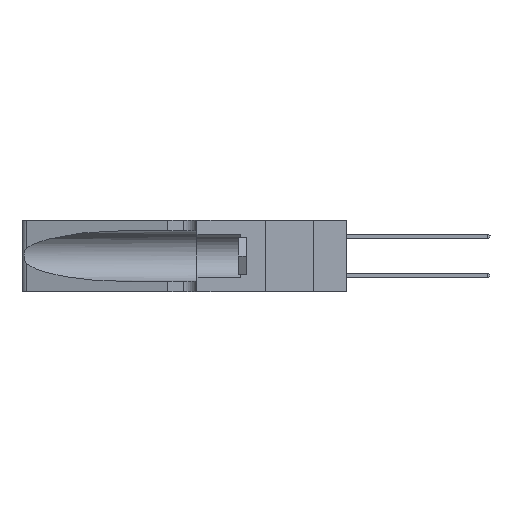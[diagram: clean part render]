
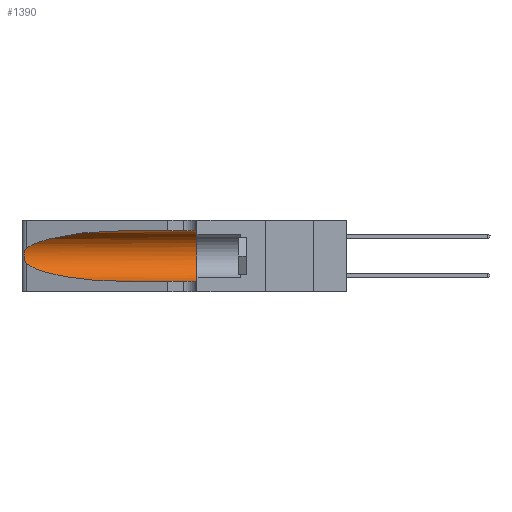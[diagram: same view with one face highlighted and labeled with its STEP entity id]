
A CAD part, left-side view. The second image highlights one B-rep face of the part: STEP entity #1390.
In plain terms, the highlighted cylindrical face has radius 3.308 mm (diameter 6.617 mm), a partial arc.
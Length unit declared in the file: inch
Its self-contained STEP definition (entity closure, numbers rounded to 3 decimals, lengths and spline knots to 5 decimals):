
#110 = CARTESIAN_POINT ( 'NONE',  ( 0.26075, 1.23896, 0.178 ) ) ;
#476 = CARTESIAN_POINT ( 'NONE',  ( 0.2373, 1.15595, 0.28018 ) ) ;
#1249 = LINE ( 'NONE', #17443, #2117 ) ;
#1390 = ADVANCED_FACE ( 'NONE', ( #17853 ), #30696, .F. ) ;
#1551 = DIRECTION ( 'NONE',  ( 0., -1., 0. ) ) ;
#2117 = VECTOR ( 'NONE', #9579, 39.37008 ) ;
#2698 = VECTOR ( 'NONE', #1551, 39.37008 ) ;
#2896 = CARTESIAN_POINT ( 'NONE',  ( 0.25856, 1.23593, 0.16098 ) ) ;
#3001 = CARTESIAN_POINT ( 'NONE',  ( 0.25487, 1.22718, 0.22369 ) ) ;
#3516 = VERTEX_POINT ( 'NONE', #25583 ) ;
#5539 = CARTESIAN_POINT ( 'NONE',  ( 0.25555, 1.22994, 0.2215 ) ) ;
#5658 = CARTESIAN_POINT ( 'NONE',  ( 0.25639, 1.23186, 0.15144 ) ) ;
#7256 = CARTESIAN_POINT ( 'NONE',  ( 0.1305, 0.72297, 0.05475 ) ) ;
#7417 = ORIENTED_EDGE ( 'NONE', *, *, #27692, .T. ) ;
#8304 = CARTESIAN_POINT ( 'NONE',  ( 0.25487, 1.22718, 0.14631 ) ) ;
#8323 = VERTEX_POINT ( 'NONE', #11542 ) ;
#8373 = CARTESIAN_POINT ( 'NONE',  ( 0.25487, 1.22718, 0.14631 ) ) ;
#8533 = B_SPLINE_CURVE_WITH_KNOTS ( 'NONE', 3,
 ( #23815, #5539, #10922, #28944, #13513, #31569, #16165, #110, #18783, #2896, #21352, #5658, #23934, #8373 ),
 .UNSPECIFIED., .F., .F.,
 ( 4, 2, 2, 2, 2, 2, 4 ),
 ( 0., 0.00027, 0.00053, 0.00107, 0.0016, 0.00187, 0.00214 ),
 .UNSPECIFIED. ) ;
#9547 = CIRCLE ( 'NONE', #22199, 0.13025 ) ;
#9579 = DIRECTION ( 'NONE',  ( 0., -1., 0. ) ) ;
#10688 = CARTESIAN_POINT ( 'NONE',  ( 0.1305, 0.35, 0.185 ) ) ;
#10922 = CARTESIAN_POINT ( 'NONE',  ( 0.25639, 1.23184, 0.21858 ) ) ;
#10957 = CARTESIAN_POINT ( 'NONE',  ( 0.18966, 0.96281, 0.05475 ) ) ;
#11426 = ORIENTED_EDGE ( 'NONE', *, *, #33828, .F. ) ;
#11542 = CARTESIAN_POINT ( 'NONE',  ( 0.1305, 0.35, 0.31525 ) ) ;
#11917 = VERTEX_POINT ( 'NONE', #7256 ) ;
#13269 = DIRECTION ( 'NONE',  ( 0., 0., 1. ) ) ;
#13513 = CARTESIAN_POINT ( 'NONE',  ( 0.25854, 1.2359, 0.20912 ) ) ;
#13858 = CARTESIAN_POINT ( 'NONE',  ( 0.1305, 0.72297, 0.31525 ) ) ;
#14127 = EDGE_CURVE ( 'NONE', #11917, #20566, #1249, .T. ) ;
#15168 = DIRECTION ( 'NONE',  ( 0., -1., 0. ) ) ;
#15667 = EDGE_LOOP ( 'NONE', ( #7417, #26430, #25985, #16263, #27397, #11426 ) ) ;
#16102 = CARTESIAN_POINT ( 'NONE',  ( 0.2373, 1.15595, 0.08982 ) ) ;
#16165 = CARTESIAN_POINT ( 'NONE',  ( 0.26075, 1.23896, 0.19203 ) ) ;
#16263 = ORIENTED_EDGE ( 'NONE', *, *, #14127, .T. ) ;
#16501 = CARTESIAN_POINT ( 'NONE',  ( 0.18966, 0.96281, 0.31525 ) ) ;
#17443 = CARTESIAN_POINT ( 'NONE',  ( 0.1305, 1.61858, 0.05475 ) ) ;
#17853 = FACE_OUTER_BOUND ( 'NONE', #15667, .T. ) ;
#18157 =( BOUNDED_CURVE ( )  B_SPLINE_CURVE ( 3, ( #13858, #16501, #476, #19125 ),
 .UNSPECIFIED., .F., .F. ) 
 B_SPLINE_CURVE_WITH_KNOTS ( ( 4, 4 ),
 ( 1.5708, 2.84003 ),
 .UNSPECIFIED. ) 
 CURVE ( )  GEOMETRIC_REPRESENTATION_ITEM ( )  RATIONAL_B_SPLINE_CURVE ( ( 1., 0.87, 0.87, 1. ) ) 
 REPRESENTATION_ITEM ( '' )  );
#18484 = LINE ( 'NONE', #30299, #2698 ) ;
#18783 = CARTESIAN_POINT ( 'NONE',  ( 0.26017, 1.23833, 0.17102 ) ) ;
#19125 = CARTESIAN_POINT ( 'NONE',  ( 0.25487, 1.22718, 0.22369 ) ) ;
#20566 = VERTEX_POINT ( 'NONE', #26972 ) ;
#20776 = AXIS2_PLACEMENT_3D ( 'NONE', #33074, #15168, #22849 ) ;
#21032 = EDGE_CURVE ( 'NONE', #28253, #3516, #8533, .T. ) ;
#21352 = CARTESIAN_POINT ( 'NONE',  ( 0.25789, 1.23486, 0.15765 ) ) ;
#22199 = AXIS2_PLACEMENT_3D ( 'NONE', #10688, #28712, #13269 ) ;
#22849 = DIRECTION ( 'NONE',  ( 0., 0., -1. ) ) ;
#23815 = CARTESIAN_POINT ( 'NONE',  ( 0.25487, 1.22718, 0.22369 ) ) ;
#23934 = CARTESIAN_POINT ( 'NONE',  ( 0.25555, 1.22993, 0.14849 ) ) ;
#24732 = EDGE_CURVE ( 'NONE', #8323, #20566, #9547, .T. ) ;
#25023 = EDGE_CURVE ( 'NONE', #3516, #11917, #30062, .T. ) ;
#25583 = CARTESIAN_POINT ( 'NONE',  ( 0.25487, 1.22718, 0.14631 ) ) ;
#25985 = ORIENTED_EDGE ( 'NONE', *, *, #25023, .T. ) ;
#26430 = ORIENTED_EDGE ( 'NONE', *, *, #21032, .T. ) ;
#26972 = CARTESIAN_POINT ( 'NONE',  ( 0.1305, 0.35, 0.05475 ) ) ;
#27397 = ORIENTED_EDGE ( 'NONE', *, *, #24732, .F. ) ;
#27692 = EDGE_CURVE ( 'NONE', #32267, #28253, #18157, .T. ) ;
#28253 = VERTEX_POINT ( 'NONE', #3001 ) ;
#28712 = DIRECTION ( 'NONE',  ( 0., 1., 0. ) ) ;
#28906 = CARTESIAN_POINT ( 'NONE',  ( 0.1305, 0.72297, 0.31525 ) ) ;
#28944 = CARTESIAN_POINT ( 'NONE',  ( 0.25787, 1.23484, 0.2124 ) ) ;
#28989 = CARTESIAN_POINT ( 'NONE',  ( 0.1305, 0.72297, 0.05475 ) ) ;
#30062 =( BOUNDED_CURVE ( )  B_SPLINE_CURVE ( 3, ( #8304, #16102, #10957, #28989 ),
 .UNSPECIFIED., .F., .F. ) 
 B_SPLINE_CURVE_WITH_KNOTS ( ( 4, 4 ),
 ( 3.44316, 4.71239 ),
 .UNSPECIFIED. ) 
 CURVE ( )  GEOMETRIC_REPRESENTATION_ITEM ( )  RATIONAL_B_SPLINE_CURVE ( ( 1., 0.87, 0.87, 1. ) ) 
 REPRESENTATION_ITEM ( '' )  );
#30299 = CARTESIAN_POINT ( 'NONE',  ( 0.1305, 1.61858, 0.31525 ) ) ;
#30696 = CYLINDRICAL_SURFACE ( 'NONE', #20776, 0.13025 ) ;
#31569 = CARTESIAN_POINT ( 'NONE',  ( 0.26018, 1.23835, 0.19895 ) ) ;
#32267 = VERTEX_POINT ( 'NONE', #28906 ) ;
#33074 = CARTESIAN_POINT ( 'NONE',  ( 0.1305, 1.61858, 0.185 ) ) ;
#33828 = EDGE_CURVE ( 'NONE', #32267, #8323, #18484, .T. ) ;
